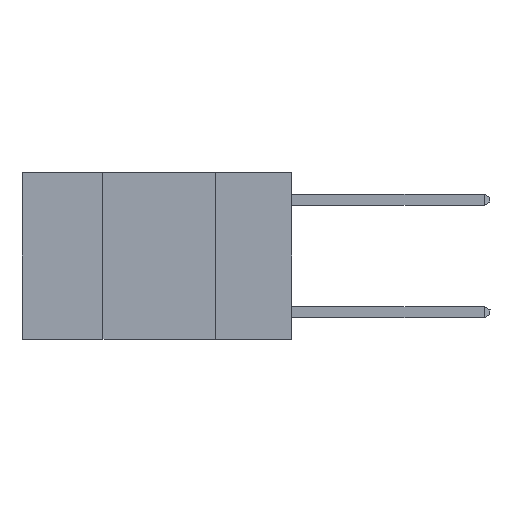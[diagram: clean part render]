
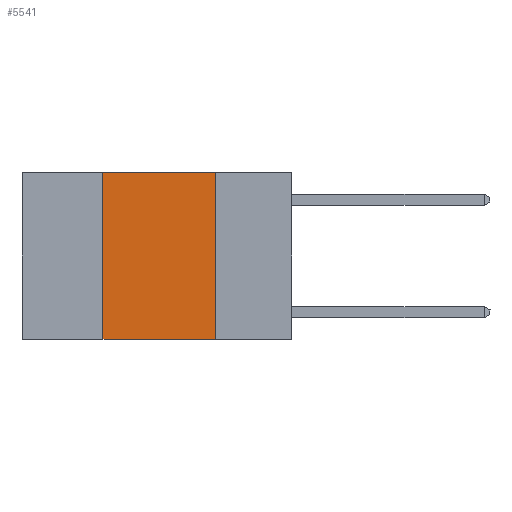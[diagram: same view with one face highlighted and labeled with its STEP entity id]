
A CAD part, left-side view. The second image highlights one B-rep face of the part: STEP entity #5541.
In plain terms, the highlighted planar face has unit normal (-1, 0, 0).
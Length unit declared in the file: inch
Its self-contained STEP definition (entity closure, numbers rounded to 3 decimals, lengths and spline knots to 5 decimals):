
#539 = VECTOR ( 'NONE', #6544, 39.37008 ) ;
#952 = PLANE ( 'NONE',  #4659 ) ;
#1011 = LINE ( 'NONE', #15124, #539 ) ;
#2055 = VECTOR ( 'NONE', #17503, 39.37008 ) ;
#2420 = DIRECTION ( 'NONE',  ( 1., 0., 0. ) ) ;
#2447 = EDGE_CURVE ( 'NONE', #16895, #10358, #9512, .T. ) ;
#2626 = LINE ( 'NONE', #9760, #17618 ) ;
#2645 = FACE_OUTER_BOUND ( 'NONE', #4541, .T. ) ;
#3725 = CARTESIAN_POINT ( 'NONE',  ( 0., 0.17, -0.37 ) ) ;
#4541 = EDGE_LOOP ( 'NONE', ( #8082, #10878, #12580, #16502 ) ) ;
#4659 = AXIS2_PLACEMENT_3D ( 'NONE', #15500, #2420, #12781 ) ;
#5091 = VERTEX_POINT ( 'NONE', #3725 ) ;
#5427 = CARTESIAN_POINT ( 'NONE',  ( 0., 0.42, -0.37 ) ) ;
#5541 = ADVANCED_FACE ( 'NONE', ( #2645 ), #952, .F. ) ;
#5897 = EDGE_CURVE ( 'NONE', #10358, #5091, #2626, .T. ) ;
#6087 = CARTESIAN_POINT ( 'NONE',  ( 0., 0.42, 0. ) ) ;
#6128 = LINE ( 'NONE', #6087, #2055 ) ;
#6544 = DIRECTION ( 'NONE',  ( 0., -1., 0. ) ) ;
#6733 = DIRECTION ( 'NONE',  ( 0., -1., 0. ) ) ;
#8082 = ORIENTED_EDGE ( 'NONE', *, *, #5897, .F. ) ;
#8335 = EDGE_CURVE ( 'NONE', #12649, #5091, #1011, .T. ) ;
#9512 = LINE ( 'NONE', #13482, #16933 ) ;
#9760 = CARTESIAN_POINT ( 'NONE',  ( 0., 0.17, 0. ) ) ;
#10358 = VERTEX_POINT ( 'NONE', #10577 ) ;
#10577 = CARTESIAN_POINT ( 'NONE',  ( 0., 0.17, 0. ) ) ;
#10878 = ORIENTED_EDGE ( 'NONE', *, *, #2447, .F. ) ;
#11165 = EDGE_CURVE ( 'NONE', #12649, #16895, #6128, .T. ) ;
#12580 = ORIENTED_EDGE ( 'NONE', *, *, #11165, .F. ) ;
#12649 = VERTEX_POINT ( 'NONE', #5427 ) ;
#12781 = DIRECTION ( 'NONE',  ( 0., 0., -1. ) ) ;
#13482 = CARTESIAN_POINT ( 'NONE',  ( 0., 0.6, 0. ) ) ;
#15124 = CARTESIAN_POINT ( 'NONE',  ( 0., 0.6, -0.37 ) ) ;
#15500 = CARTESIAN_POINT ( 'NONE',  ( 0., 0.6, 0. ) ) ;
#16502 = ORIENTED_EDGE ( 'NONE', *, *, #8335, .T. ) ;
#16895 = VERTEX_POINT ( 'NONE', #18308 ) ;
#16933 = VECTOR ( 'NONE', #6733, 39.37008 ) ;
#17503 = DIRECTION ( 'NONE',  ( 0., 0., 1. ) ) ;
#17618 = VECTOR ( 'NONE', #18112, 39.37008 ) ;
#18112 = DIRECTION ( 'NONE',  ( 0., 0., -1. ) ) ;
#18308 = CARTESIAN_POINT ( 'NONE',  ( 0., 0.42, 0. ) ) ;
